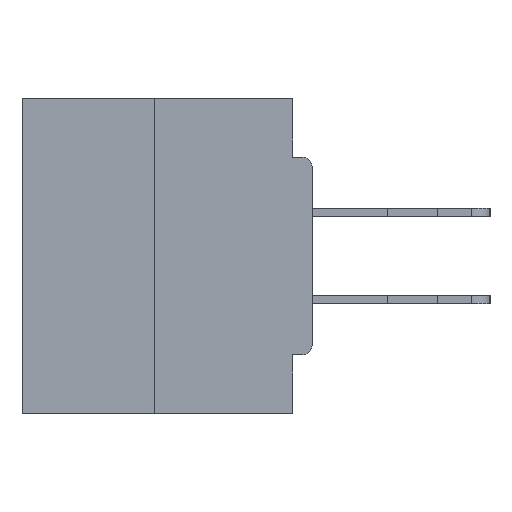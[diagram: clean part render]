
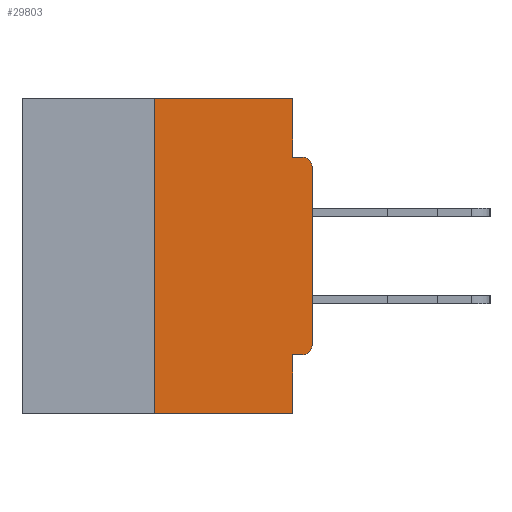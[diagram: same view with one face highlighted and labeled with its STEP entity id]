
A CAD part, left-side view. The second image highlights one B-rep face of the part: STEP entity #29803.
In plain terms, the highlighted planar face has unit normal (-1, 0, 0).
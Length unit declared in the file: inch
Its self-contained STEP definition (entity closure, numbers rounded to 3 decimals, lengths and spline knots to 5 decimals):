
#190 = ORIENTED_EDGE ( 'NONE', *, *, #2614, .T. ) ;
#595 = AXIS2_PLACEMENT_3D ( 'NONE', #13834, #33287, #19439 ) ;
#648 = CARTESIAN_POINT ( 'NONE',  ( 0., 0., 0. ) ) ;
#1328 = LINE ( 'NONE', #29752, #25726 ) ;
#1745 = EDGE_CURVE ( 'NONE', #35264, #12422, #6304, .T. ) ;
#1941 = VERTEX_POINT ( 'NONE', #8557 ) ;
#2609 = DIRECTION ( 'NONE',  ( 0., 0., -1. ) ) ;
#2614 = EDGE_CURVE ( 'NONE', #35935, #23715, #16222, .T. ) ;
#2966 = CARTESIAN_POINT ( 'NONE',  ( 0., 0.031, -0.4065 ) ) ;
#3371 = EDGE_LOOP ( 'NONE', ( #4033, #16733, #190, #4499, #11686, #28171, #5470, #7578, #5276, #12860 ) ) ;
#3509 = DIRECTION ( 'NONE',  ( 1., 0., 0. ) ) ;
#3914 = CARTESIAN_POINT ( 'NONE',  ( 0., 0., -0.0935 ) ) ;
#4030 = CARTESIAN_POINT ( 'NONE',  ( 0., 0.46, -0.5 ) ) ;
#4033 = ORIENTED_EDGE ( 'NONE', *, *, #21124, .F. ) ;
#4499 = ORIENTED_EDGE ( 'NONE', *, *, #25527, .F. ) ;
#5082 = CARTESIAN_POINT ( 'NONE',  ( 0., 0.031, -0.5 ) ) ;
#5276 = ORIENTED_EDGE ( 'NONE', *, *, #5389, .F. ) ;
#5389 = EDGE_CURVE ( 'NONE', #27493, #8780, #24279, .T. ) ;
#5470 = ORIENTED_EDGE ( 'NONE', *, *, #25784, .T. ) ;
#6304 = LINE ( 'NONE', #29394, #19367 ) ;
#6646 = DIRECTION ( 'NONE',  ( 0., 0., 1. ) ) ;
#6756 = DIRECTION ( 'NONE',  ( 0., -1., 0. ) ) ;
#6845 = CARTESIAN_POINT ( 'NONE',  ( 0., 0.015, -0.0935 ) ) ;
#7031 = CARTESIAN_POINT ( 'NONE',  ( 0., 0.015, -0.4065 ) ) ;
#7050 = DIRECTION ( 'NONE',  ( 0., 0., -1. ) ) ;
#7578 = ORIENTED_EDGE ( 'NONE', *, *, #10683, .T. ) ;
#8412 = VECTOR ( 'NONE', #34299, 39.37008 ) ;
#8557 = CARTESIAN_POINT ( 'NONE',  ( 0., 0.031, 0. ) ) ;
#8780 = VERTEX_POINT ( 'NONE', #6845 ) ;
#9427 = CARTESIAN_POINT ( 'NONE',  ( 0., 0.46, 0. ) ) ;
#9483 = CARTESIAN_POINT ( 'NONE',  ( 0., 0.015, -0.1085 ) ) ;
#10027 = CARTESIAN_POINT ( 'NONE',  ( 0., 0.25, -0.5 ) ) ;
#10683 = EDGE_CURVE ( 'NONE', #16857, #8780, #35441, .T. ) ;
#11017 = VECTOR ( 'NONE', #6756, 39.37008 ) ;
#11040 = LINE ( 'NONE', #25801, #8412 ) ;
#11686 = ORIENTED_EDGE ( 'NONE', *, *, #1745, .F. ) ;
#11920 = CARTESIAN_POINT ( 'NONE',  ( 0., 0.46, 0. ) ) ;
#12205 = CARTESIAN_POINT ( 'NONE',  ( 0., 0.031, -0.0935 ) ) ;
#12422 = VERTEX_POINT ( 'NONE', #2966 ) ;
#12860 = ORIENTED_EDGE ( 'NONE', *, *, #35350, .F. ) ;
#12874 = DIRECTION ( 'NONE',  ( 0., 0., -1. ) ) ;
#13024 = EDGE_CURVE ( 'NONE', #35935, #33039, #11040, .T. ) ;
#13587 = VERTEX_POINT ( 'NONE', #19503 ) ;
#13731 = AXIS2_PLACEMENT_3D ( 'NONE', #9427, #3509, #34572 ) ;
#13834 = CARTESIAN_POINT ( 'NONE',  ( 0., 0.015, -0.3915 ) ) ;
#16222 = LINE ( 'NONE', #4030, #11017 ) ;
#16733 = ORIENTED_EDGE ( 'NONE', *, *, #13024, .F. ) ;
#16857 = VERTEX_POINT ( 'NONE', #33694 ) ;
#16884 = VECTOR ( 'NONE', #29358, 39.37008 ) ;
#17639 = DIRECTION ( 'NONE',  ( 0., -1., 0. ) ) ;
#18159 = VECTOR ( 'NONE', #6646, 39.37008 ) ;
#19367 = VECTOR ( 'NONE', #26607, 39.37008 ) ;
#19439 = DIRECTION ( 'NONE',  ( 0., 0., -1. ) ) ;
#19503 = CARTESIAN_POINT ( 'NONE',  ( 0., 0., -0.3915 ) ) ;
#20359 = VECTOR ( 'NONE', #17639, 39.37008 ) ;
#21124 = EDGE_CURVE ( 'NONE', #33039, #1941, #24274, .T. ) ;
#22240 = FACE_OUTER_BOUND ( 'NONE', #3371, .T. ) ;
#22916 = LINE ( 'NONE', #648, #18159 ) ;
#22942 = VECTOR ( 'NONE', #2609, 39.37008 ) ;
#23206 = CIRCLE ( 'NONE', #595, 0.015 ) ;
#23259 = EDGE_CURVE ( 'NONE', #35264, #13587, #23206, .T. ) ;
#23284 = PLANE ( 'NONE',  #13731 ) ;
#23715 = VERTEX_POINT ( 'NONE', #31620 ) ;
#24274 = LINE ( 'NONE', #11920, #20359 ) ;
#24279 = LINE ( 'NONE', #3914, #16884 ) ;
#25527 = EDGE_CURVE ( 'NONE', #12422, #23715, #29903, .T. ) ;
#25726 = VECTOR ( 'NONE', #12874, 39.37008 ) ;
#25784 = EDGE_CURVE ( 'NONE', #13587, #16857, #22916, .T. ) ;
#25801 = CARTESIAN_POINT ( 'NONE',  ( 0., 0.25, 0. ) ) ;
#26607 = DIRECTION ( 'NONE',  ( 0., 1., 0. ) ) ;
#27493 = VERTEX_POINT ( 'NONE', #12205 ) ;
#28171 = ORIENTED_EDGE ( 'NONE', *, *, #23259, .T. ) ;
#29358 = DIRECTION ( 'NONE',  ( 0., -1., 0. ) ) ;
#29394 = CARTESIAN_POINT ( 'NONE',  ( 0., 0., -0.4065 ) ) ;
#29752 = CARTESIAN_POINT ( 'NONE',  ( 0., 0.031, 0. ) ) ;
#29803 = ADVANCED_FACE ( 'NONE', ( #22240 ), #23284, .F. ) ;
#29903 = LINE ( 'NONE', #5082, #22942 ) ;
#31620 = CARTESIAN_POINT ( 'NONE',  ( 0., 0.031, -0.5 ) ) ;
#31722 = DIRECTION ( 'NONE',  ( -1., 0., 0. ) ) ;
#33039 = VERTEX_POINT ( 'NONE', #35998 ) ;
#33287 = DIRECTION ( 'NONE',  ( -1., 0., 0. ) ) ;
#33694 = CARTESIAN_POINT ( 'NONE',  ( 0., 0., -0.1085 ) ) ;
#34299 = DIRECTION ( 'NONE',  ( 0., 0., 1. ) ) ;
#34572 = DIRECTION ( 'NONE',  ( 0., 0., -1. ) ) ;
#34875 = AXIS2_PLACEMENT_3D ( 'NONE', #9483, #31722, #7050 ) ;
#35264 = VERTEX_POINT ( 'NONE', #7031 ) ;
#35350 = EDGE_CURVE ( 'NONE', #1941, #27493, #1328, .T. ) ;
#35441 = CIRCLE ( 'NONE', #34875, 0.015 ) ;
#35935 = VERTEX_POINT ( 'NONE', #10027 ) ;
#35998 = CARTESIAN_POINT ( 'NONE',  ( 0., 0.25, 0. ) ) ;
